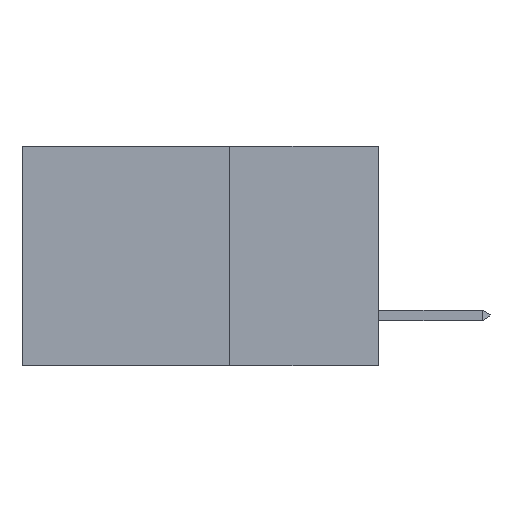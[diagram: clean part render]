
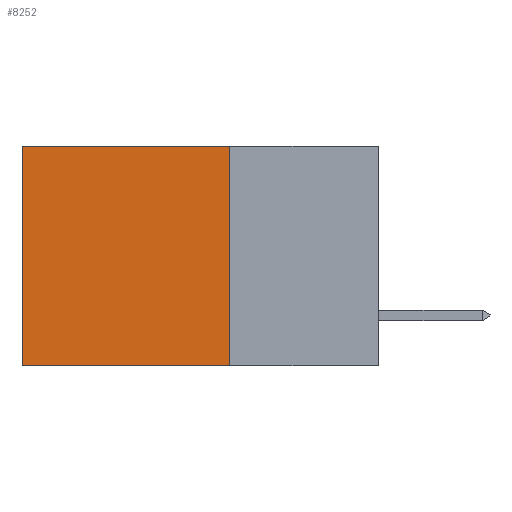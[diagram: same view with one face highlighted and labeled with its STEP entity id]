
A CAD part, left-side view. The second image highlights one B-rep face of the part: STEP entity #8252.
In plain terms, the highlighted planar face has unit normal (-1, 0, 0).
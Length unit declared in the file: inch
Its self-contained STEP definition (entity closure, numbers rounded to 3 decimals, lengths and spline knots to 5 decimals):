
#44 = EDGE_CURVE ( 'NONE', #5358, #6422, #2436, .T. ) ;
#264 = ORIENTED_EDGE ( 'NONE', *, *, #44, .F. ) ;
#529 = CARTESIAN_POINT ( 'NONE',  ( 0.298, 0.6, 0. ) ) ;
#797 = CARTESIAN_POINT ( 'NONE',  ( 0.298, 0.25, 0. ) ) ;
#1440 = LINE ( 'NONE', #797, #3074 ) ;
#1568 = DIRECTION ( 'NONE',  ( 0., 0., -1. ) ) ;
#1880 = CARTESIAN_POINT ( 'NONE',  ( 0.298, 0.25, -0.37 ) ) ;
#2115 = AXIS2_PLACEMENT_3D ( 'NONE', #10609, #11519, #1568 ) ;
#2436 = LINE ( 'NONE', #1880, #9800 ) ;
#2450 = EDGE_LOOP ( 'NONE', ( #7881, #264, #5508, #10522 ) ) ;
#2936 = EDGE_CURVE ( 'NONE', #10624, #6183, #1440, .T. ) ;
#3074 = VECTOR ( 'NONE', #8805, 39.37008 ) ;
#3667 = DIRECTION ( 'NONE',  ( 0., 1., 0. ) ) ;
#4199 = CARTESIAN_POINT ( 'NONE',  ( 0.298, 0.25, 0. ) ) ;
#4241 = PLANE ( 'NONE',  #2115 ) ;
#4473 = EDGE_CURVE ( 'NONE', #10624, #5358, #6018, .T. ) ;
#5358 = VERTEX_POINT ( 'NONE', #7403 ) ;
#5508 = ORIENTED_EDGE ( 'NONE', *, *, #4473, .F. ) ;
#5730 = VECTOR ( 'NONE', #10632, 39.37008 ) ;
#6018 = LINE ( 'NONE', #7139, #5730 ) ;
#6183 = VERTEX_POINT ( 'NONE', #529 ) ;
#6422 = VERTEX_POINT ( 'NONE', #11437 ) ;
#7139 = CARTESIAN_POINT ( 'NONE',  ( 0.298, 0.25, 0. ) ) ;
#7403 = CARTESIAN_POINT ( 'NONE',  ( 0.298, 0.25, -0.37 ) ) ;
#7881 = ORIENTED_EDGE ( 'NONE', *, *, #10237, .T. ) ;
#8252 = ADVANCED_FACE ( 'NONE', ( #9029 ), #4241, .F. ) ;
#8289 = LINE ( 'NONE', #8826, #8710 ) ;
#8710 = VECTOR ( 'NONE', #11569, 39.37008 ) ;
#8805 = DIRECTION ( 'NONE',  ( 0., 1., 0. ) ) ;
#8826 = CARTESIAN_POINT ( 'NONE',  ( 0.298, 0.6, 0. ) ) ;
#9029 = FACE_OUTER_BOUND ( 'NONE', #2450, .T. ) ;
#9800 = VECTOR ( 'NONE', #3667, 39.37008 ) ;
#10237 = EDGE_CURVE ( 'NONE', #6183, #6422, #8289, .T. ) ;
#10522 = ORIENTED_EDGE ( 'NONE', *, *, #2936, .T. ) ;
#10609 = CARTESIAN_POINT ( 'NONE',  ( 0.298, 0.25, 0. ) ) ;
#10624 = VERTEX_POINT ( 'NONE', #4199 ) ;
#10632 = DIRECTION ( 'NONE',  ( 0., 0., -1. ) ) ;
#11437 = CARTESIAN_POINT ( 'NONE',  ( 0.298, 0.6, -0.37 ) ) ;
#11519 = DIRECTION ( 'NONE',  ( 1., 0., 0. ) ) ;
#11569 = DIRECTION ( 'NONE',  ( 0., 0., -1. ) ) ;
